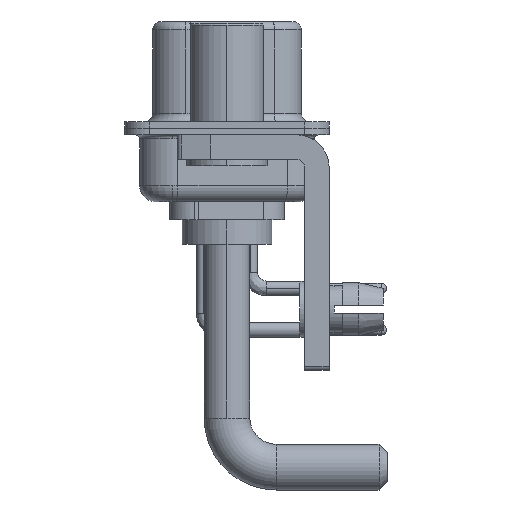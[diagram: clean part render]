
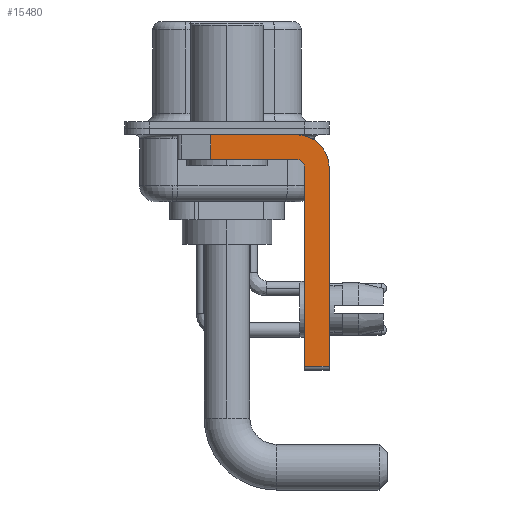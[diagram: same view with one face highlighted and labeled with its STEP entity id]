
A CAD part, left-side view. The second image highlights one B-rep face of the part: STEP entity #15480.
In plain terms, the highlighted planar face has unit normal (-1, 0, 0).
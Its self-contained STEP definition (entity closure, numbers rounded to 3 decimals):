
#997 = PLANE ( 'NONE',  #17050 ) ;
#1302 = DIRECTION ( 'NONE',  ( -1., 0., 0. ) ) ;
#1304 = DIRECTION ( 'NONE',  ( 0., -1., 0. ) ) ;
#1482 = EDGE_CURVE ( 'NONE', #26962, #14300, #16825, .T. ) ;
#1631 = DIRECTION ( 'NONE',  ( 0., 0., -1. ) ) ;
#1890 = CARTESIAN_POINT ( 'NONE',  ( -2.9, -4.25, -2.4 ) ) ;
#2007 = VERTEX_POINT ( 'NONE', #22086 ) ;
#4271 = LINE ( 'NONE', #14014, #17649 ) ;
#5127 = CARTESIAN_POINT ( 'NONE',  ( -2.9, -6.25, -2.4 ) ) ;
#5149 = EDGE_CURVE ( 'NONE', #15436, #2007, #4271, .T. ) ;
#5152 = EDGE_CURVE ( 'NONE', #19630, #13042, #13102, .T. ) ;
#5909 = ORIENTED_EDGE ( 'NONE', *, *, #9237, .F. ) ;
#6000 = VERTEX_POINT ( 'NONE', #7782 ) ;
#6461 = CARTESIAN_POINT ( 'NONE',  ( -2.9, -4.75, -14.55 ) ) ;
#6594 = DIRECTION ( 'NONE',  ( 0., 0., -1. ) ) ;
#6896 = DIRECTION ( 'NONE',  ( 0., 0., 1. ) ) ;
#7329 = VECTOR ( 'NONE', #14296, 1000. ) ;
#7782 = CARTESIAN_POINT ( 'NONE',  ( -2.9, -4.25, -1.9 ) ) ;
#7837 = EDGE_CURVE ( 'NONE', #20675, #6000, #30612, .T. ) ;
#7877 = VECTOR ( 'NONE', #1304, 1000. ) ;
#8511 = LINE ( 'NONE', #18660, #7877 ) ;
#9237 = EDGE_CURVE ( 'NONE', #13042, #2007, #18671, .T. ) ;
#9523 = ORIENTED_EDGE ( 'NONE', *, *, #5149, .T. ) ;
#9928 = ORIENTED_EDGE ( 'NONE', *, *, #1482, .T. ) ;
#11051 = DIRECTION ( 'NONE',  ( 0., 0., 1. ) ) ;
#11344 = CARTESIAN_POINT ( 'NONE',  ( -2.9, -4.25, -2.4 ) ) ;
#11457 = ORIENTED_EDGE ( 'NONE', *, *, #14519, .F. ) ;
#12542 = DIRECTION ( 'NONE',  ( 0., 1., 0. ) ) ;
#13042 = VERTEX_POINT ( 'NONE', #5127 ) ;
#13102 = CIRCLE ( 'NONE', #29823, 2. ) ;
#13282 = VECTOR ( 'NONE', #6896, 1000. ) ;
#14014 = CARTESIAN_POINT ( 'NONE',  ( -2.9, -4.25, -14.55 ) ) ;
#14122 = ORIENTED_EDGE ( 'NONE', *, *, #29863, .F. ) ;
#14296 = DIRECTION ( 'NONE',  ( 0., 0., -1. ) ) ;
#14300 = VERTEX_POINT ( 'NONE', #17559 ) ;
#14519 = EDGE_CURVE ( 'NONE', #26962, #19630, #8511, .T. ) ;
#14676 = ORIENTED_EDGE ( 'NONE', *, *, #7837, .F. ) ;
#14853 = VECTOR ( 'NONE', #6594, 1000. ) ;
#15117 = CARTESIAN_POINT ( 'NONE',  ( -2.9, 0.978, -0.4 ) ) ;
#15436 = VERTEX_POINT ( 'NONE', #6461 ) ;
#15480 = ADVANCED_FACE ( 'NONE', ( #20417 ), #997, .F. ) ;
#16825 = LINE ( 'NONE', #21750, #7329 ) ;
#16977 = CARTESIAN_POINT ( 'NONE',  ( -2.9, -4.25, -1.9 ) ) ;
#17050 = AXIS2_PLACEMENT_3D ( 'NONE', #23447, #30760, #1631 ) ;
#17153 = ORIENTED_EDGE ( 'NONE', *, *, #19834, .F. ) ;
#17559 = CARTESIAN_POINT ( 'NONE',  ( -2.9, 0.978, -1.9 ) ) ;
#17565 = VECTOR ( 'NONE', #12542, 1000. ) ;
#17649 = VECTOR ( 'NONE', #23684, 1000. ) ;
#18516 = EDGE_LOOP ( 'NONE', ( #11457, #9928, #17153, #14676, #14122, #9523, #5909, #29390 ) ) ;
#18660 = CARTESIAN_POINT ( 'NONE',  ( -2.9, 3., -0.4 ) ) ;
#18671 = LINE ( 'NONE', #28363, #14853 ) ;
#18908 = DIRECTION ( 'NONE',  ( 1., 0., 0. ) ) ;
#18963 = LINE ( 'NONE', #19132, #13282 ) ;
#19132 = CARTESIAN_POINT ( 'NONE',  ( -2.9, -4.75, -14.8 ) ) ;
#19630 = VERTEX_POINT ( 'NONE', #25274 ) ;
#19834 = EDGE_CURVE ( 'NONE', #6000, #14300, #28902, .T. ) ;
#20417 = FACE_OUTER_BOUND ( 'NONE', #18516, .T. ) ;
#20675 = VERTEX_POINT ( 'NONE', #25095 ) ;
#21750 = CARTESIAN_POINT ( 'NONE',  ( -2.9, 0.978, -1.9 ) ) ;
#22086 = CARTESIAN_POINT ( 'NONE',  ( -2.9, -6.25, -14.55 ) ) ;
#22994 = AXIS2_PLACEMENT_3D ( 'NONE', #11344, #1302, #11051 ) ;
#23447 = CARTESIAN_POINT ( 'NONE',  ( -2.9, -4.25, -2.4 ) ) ;
#23684 = DIRECTION ( 'NONE',  ( 0., -1., 0. ) ) ;
#25095 = CARTESIAN_POINT ( 'NONE',  ( -2.9, -4.75, -2.4 ) ) ;
#25274 = CARTESIAN_POINT ( 'NONE',  ( -2.9, -4.25, -0.4 ) ) ;
#26962 = VERTEX_POINT ( 'NONE', #15117 ) ;
#28363 = CARTESIAN_POINT ( 'NONE',  ( -2.9, -6.25, -2.4 ) ) ;
#28598 = DIRECTION ( 'NONE',  ( 0., 0., -1. ) ) ;
#28902 = LINE ( 'NONE', #16977, #17565 ) ;
#29390 = ORIENTED_EDGE ( 'NONE', *, *, #5152, .F. ) ;
#29823 = AXIS2_PLACEMENT_3D ( 'NONE', #1890, #18908, #28598 ) ;
#29863 = EDGE_CURVE ( 'NONE', #15436, #20675, #18963, .T. ) ;
#30612 = CIRCLE ( 'NONE', #22994, 0.5 ) ;
#30760 = DIRECTION ( 'NONE',  ( 1., 0., 0. ) ) ;
